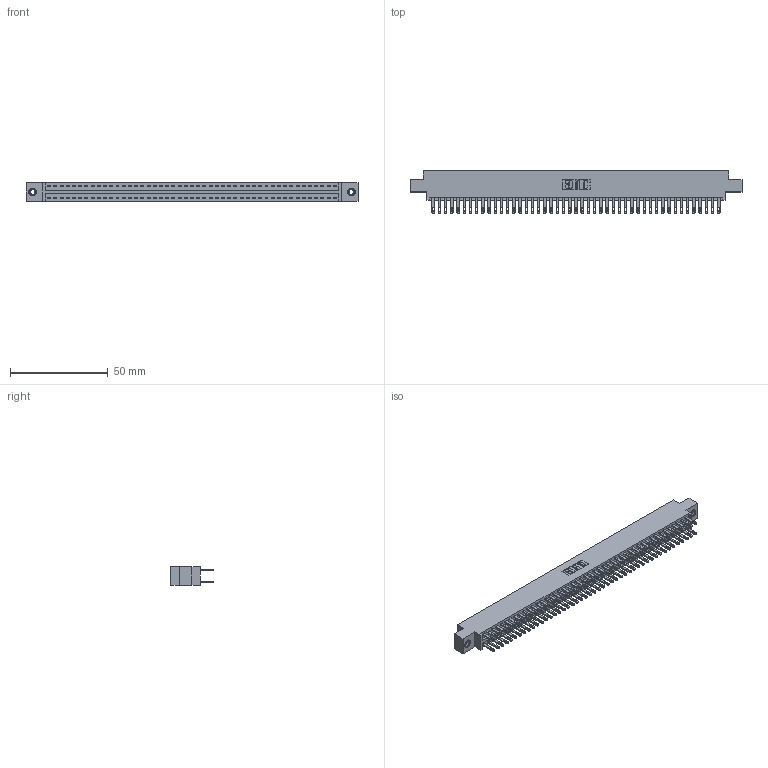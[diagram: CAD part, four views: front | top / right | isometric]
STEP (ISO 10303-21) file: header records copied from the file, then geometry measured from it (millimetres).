
FILE_DESCRIPTION (( 'STEP AP203' ), '1' );
FILE_NAME ('346-094-500-807.STEP', '2022-05-26T09:11:39', ( '' ), ( '' ), 'SwSTEP 2.0', 'SolidWorks 2020', '' );
FILE_SCHEMA (( 'CONFIG_CONTROL_DESIGN' ));
Length unit declared in the file: inch
Products named in the file (4): 345-292-001_345-293-100; 346 Part_0.170 Offset - 0.156 Dia-TI; 346-094-500-807; 345-250-001_345-250-005-103
Assembly tree (97 placements, depth 2):
  346-094-500-807
    346 Part_0.170 Offset - 0.156 Dia-TI
    345-292-001_345-293-100  x94
    345-250-001_345-250-005-103  x2
Bounding box: 169.8 x 21.84 x 9.4 mm (x, y, z)
Volume: 16715.5 mm3; surface area: 24252.3 mm2
Topology: 97 solids, 97 shells, 4698 faces, 14295 edges, 9522 vertices
Faces by surface type: plane 2838, cylinder 1844, cone 12, torus 4
Entity records: 31248 total; most frequent: CARTESIAN_POINT 5127, ORIENTED_EDGE 5054, DIRECTION 4597, EDGE_CURVE 2527, VECTOR 2183, LINE 2183, VERTEX_POINT 1680, AXIS2_PLACEMENT_3D 1207
